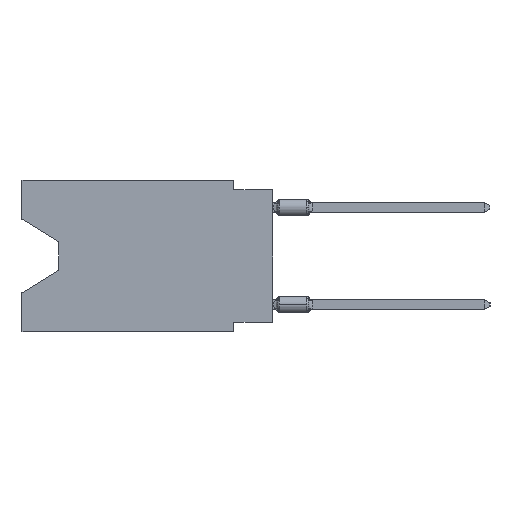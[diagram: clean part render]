
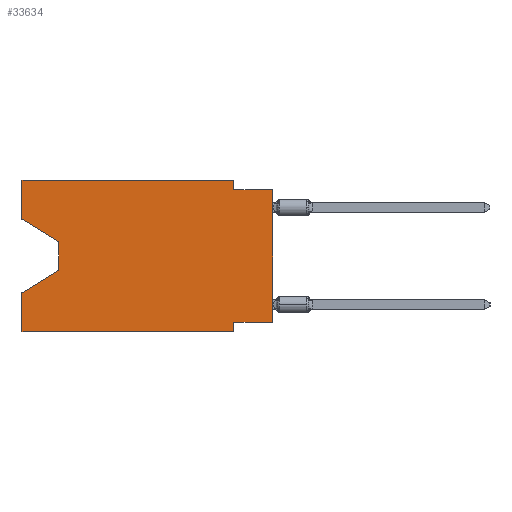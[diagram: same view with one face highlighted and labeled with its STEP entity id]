
A CAD part, left-side view. The second image highlights one B-rep face of the part: STEP entity #33634.
In plain terms, the highlighted planar face has unit normal (-1, 0, 0).
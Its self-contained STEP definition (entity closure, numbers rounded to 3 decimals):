
#579 = EDGE_CURVE ( 'NONE', #60065, #9687, #6288, .T. ) ;
#953 = CARTESIAN_POINT ( 'NONE',  ( 0., 13.97, -5.893 ) ) ;
#1738 = ORIENTED_EDGE ( 'NONE', *, *, #60788, .T. ) ;
#1933 = EDGE_CURVE ( 'NONE', #21924, #43712, #15814, .T. ) ;
#2366 = VERTEX_POINT ( 'NONE', #20881 ) ;
#2608 = VECTOR ( 'NONE', #40500, 1000. ) ;
#2714 = EDGE_CURVE ( 'NONE', #6544, #10024, #42644, .T. ) ;
#2910 = LINE ( 'NONE', #50467, #2608 ) ;
#3443 = LINE ( 'NONE', #23006, #52437 ) ;
#3697 = ORIENTED_EDGE ( 'NONE', *, *, #2714, .T. ) ;
#5980 = LINE ( 'NONE', #60244, #28056 ) ;
#6183 = CARTESIAN_POINT ( 'NONE',  ( 0., 2.54, 0. ) ) ;
#6288 = LINE ( 'NONE', #57298, #52008 ) ;
#6544 = VERTEX_POINT ( 'NONE', #12046 ) ;
#7471 = ORIENTED_EDGE ( 'NONE', *, *, #1933, .F. ) ;
#8336 = CARTESIAN_POINT ( 'NONE',  ( 0., 13.97, -5.893 ) ) ;
#8692 = VERTEX_POINT ( 'NONE', #8336 ) ;
#9005 = LINE ( 'NONE', #23456, #18181 ) ;
#9687 = VERTEX_POINT ( 'NONE', #48682 ) ;
#10024 = VERTEX_POINT ( 'NONE', #12346 ) ;
#10791 = CARTESIAN_POINT ( 'NONE',  ( 0., 0., -0.635 ) ) ;
#10817 = DIRECTION ( 'NONE',  ( 0., 0., 1. ) ) ;
#12046 = CARTESIAN_POINT ( 'NONE',  ( 0., 0., -9.271 ) ) ;
#12173 = VECTOR ( 'NONE', #49851, 1000. ) ;
#12346 = CARTESIAN_POINT ( 'NONE',  ( 0., 0., -0.635 ) ) ;
#12454 = VECTOR ( 'NONE', #60430, 1000. ) ;
#12870 = DIRECTION ( 'NONE',  ( 0., 0., 1. ) ) ;
#13050 = CARTESIAN_POINT ( 'NONE',  ( 0., 2.54, -9.271 ) ) ;
#13128 = ORIENTED_EDGE ( 'NONE', *, *, #51989, .T. ) ;
#14111 = EDGE_CURVE ( 'NONE', #6544, #60065, #21575, .T. ) ;
#14609 = DIRECTION ( 'NONE',  ( 1., 0., 0. ) ) ;
#14720 = AXIS2_PLACEMENT_3D ( 'NONE', #19420, #14609, #38994 ) ;
#15311 = VECTOR ( 'NONE', #25221, 1000. ) ;
#15359 = EDGE_LOOP ( 'NONE', ( #57547, #1738, #18326, #15577, #13128, #36729, #48830, #3697, #20250, #7471, #39757, #35661 ) ) ;
#15577 = ORIENTED_EDGE ( 'NONE', *, *, #54805, .F. ) ;
#15814 = LINE ( 'NONE', #6183, #12173 ) ;
#16882 = VECTOR ( 'NONE', #25194, 1000. ) ;
#17062 = CARTESIAN_POINT ( 'NONE',  ( 0., 16.383, 0. ) ) ;
#17173 = DIRECTION ( 'NONE',  ( 0., 0., -1. ) ) ;
#18181 = VECTOR ( 'NONE', #28917, 1000. ) ;
#18326 = ORIENTED_EDGE ( 'NONE', *, *, #41198, .T. ) ;
#19420 = CARTESIAN_POINT ( 'NONE',  ( 0., 16.383, 0. ) ) ;
#20098 = LINE ( 'NONE', #10791, #15311 ) ;
#20250 = ORIENTED_EDGE ( 'NONE', *, *, #63071, .F. ) ;
#20881 = CARTESIAN_POINT ( 'NONE',  ( 0., 16.383, -2.546 ) ) ;
#21154 = DIRECTION ( 'NONE',  ( 0., 0.855, -0.519 ) ) ;
#21252 = CARTESIAN_POINT ( 'NONE',  ( 0., 0., -9.271 ) ) ;
#21575 = LINE ( 'NONE', #21252, #12454 ) ;
#21924 = VERTEX_POINT ( 'NONE', #59387 ) ;
#23006 = CARTESIAN_POINT ( 'NONE',  ( 0., 16.383, -9.906 ) ) ;
#23456 = CARTESIAN_POINT ( 'NONE',  ( 0., 13.97, -4.013 ) ) ;
#23921 = FACE_OUTER_BOUND ( 'NONE', #15359, .T. ) ;
#25194 = DIRECTION ( 'NONE',  ( 0., -1., 0. ) ) ;
#25221 = DIRECTION ( 'NONE',  ( 0., -1., 0. ) ) ;
#25337 = CARTESIAN_POINT ( 'NONE',  ( 0., 16.383, -9.906 ) ) ;
#26370 = CARTESIAN_POINT ( 'NONE',  ( 0., 13.97, -4.013 ) ) ;
#28056 = VECTOR ( 'NONE', #10817, 1000. ) ;
#28917 = DIRECTION ( 'NONE',  ( 0., 0., -1. ) ) ;
#29521 = VERTEX_POINT ( 'NONE', #60179 ) ;
#30034 = CARTESIAN_POINT ( 'NONE',  ( 0., 16.383, 0. ) ) ;
#33634 = ADVANCED_FACE ( 'NONE', ( #23921 ), #43501, .F. ) ;
#35478 = EDGE_CURVE ( 'NONE', #2366, #29521, #56545, .T. ) ;
#35661 = ORIENTED_EDGE ( 'NONE', *, *, #35478, .F. ) ;
#36729 = ORIENTED_EDGE ( 'NONE', *, *, #579, .F. ) ;
#36756 = VERTEX_POINT ( 'NONE', #26370 ) ;
#36833 = EDGE_CURVE ( 'NONE', #2366, #36756, #2910, .T. ) ;
#38994 = DIRECTION ( 'NONE',  ( 0., 0., -1. ) ) ;
#39757 = ORIENTED_EDGE ( 'NONE', *, *, #57748, .F. ) ;
#39765 = LINE ( 'NONE', #953, #42818 ) ;
#40500 = DIRECTION ( 'NONE',  ( 0., -0.855, -0.519 ) ) ;
#41198 = EDGE_CURVE ( 'NONE', #8692, #49334, #39765, .T. ) ;
#42579 = DIRECTION ( 'NONE',  ( 0., -1., 0. ) ) ;
#42644 = LINE ( 'NONE', #62230, #57406 ) ;
#42818 = VECTOR ( 'NONE', #21154, 1000. ) ;
#43501 = PLANE ( 'NONE',  #14720 ) ;
#43634 = VERTEX_POINT ( 'NONE', #25337 ) ;
#43712 = VERTEX_POINT ( 'NONE', #58438 ) ;
#44152 = LINE ( 'NONE', #30034, #16882 ) ;
#48682 = CARTESIAN_POINT ( 'NONE',  ( 0., 2.54, -9.906 ) ) ;
#48830 = ORIENTED_EDGE ( 'NONE', *, *, #14111, .F. ) ;
#49334 = VERTEX_POINT ( 'NONE', #50872 ) ;
#49851 = DIRECTION ( 'NONE',  ( 0., 0., -1. ) ) ;
#50467 = CARTESIAN_POINT ( 'NONE',  ( 0., 16.383, -2.546 ) ) ;
#50872 = CARTESIAN_POINT ( 'NONE',  ( 0., 16.383, -7.36 ) ) ;
#51989 = EDGE_CURVE ( 'NONE', #43634, #9687, #3443, .T. ) ;
#52008 = VECTOR ( 'NONE', #17173, 1000. ) ;
#52437 = VECTOR ( 'NONE', #42579, 1000. ) ;
#54522 = DIRECTION ( 'NONE',  ( 0., 0., 1. ) ) ;
#54805 = EDGE_CURVE ( 'NONE', #43634, #49334, #5980, .T. ) ;
#56545 = LINE ( 'NONE', #17062, #59953 ) ;
#57298 = CARTESIAN_POINT ( 'NONE',  ( 0., 2.54, -9.906 ) ) ;
#57406 = VECTOR ( 'NONE', #54522, 1000. ) ;
#57547 = ORIENTED_EDGE ( 'NONE', *, *, #36833, .T. ) ;
#57748 = EDGE_CURVE ( 'NONE', #29521, #21924, #44152, .T. ) ;
#58438 = CARTESIAN_POINT ( 'NONE',  ( 0., 2.54, -0.635 ) ) ;
#59387 = CARTESIAN_POINT ( 'NONE',  ( 0., 2.54, 0. ) ) ;
#59953 = VECTOR ( 'NONE', #12870, 1000. ) ;
#60065 = VERTEX_POINT ( 'NONE', #13050 ) ;
#60179 = CARTESIAN_POINT ( 'NONE',  ( 0., 16.383, 0. ) ) ;
#60244 = CARTESIAN_POINT ( 'NONE',  ( 0., 16.383, 0. ) ) ;
#60430 = DIRECTION ( 'NONE',  ( 0., 1., 0. ) ) ;
#60788 = EDGE_CURVE ( 'NONE', #36756, #8692, #9005, .T. ) ;
#62230 = CARTESIAN_POINT ( 'NONE',  ( 0., 0., 0. ) ) ;
#63071 = EDGE_CURVE ( 'NONE', #43712, #10024, #20098, .T. ) ;
